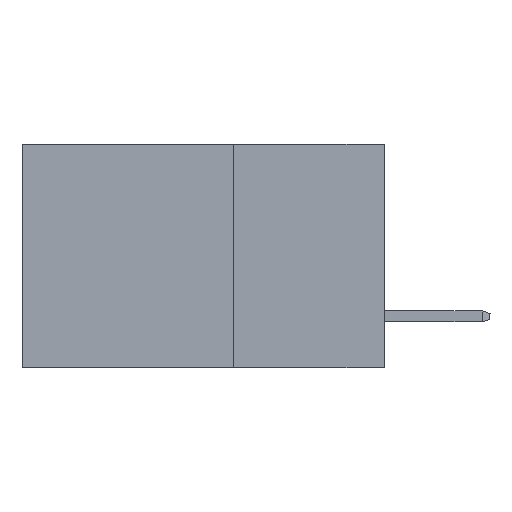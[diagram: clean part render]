
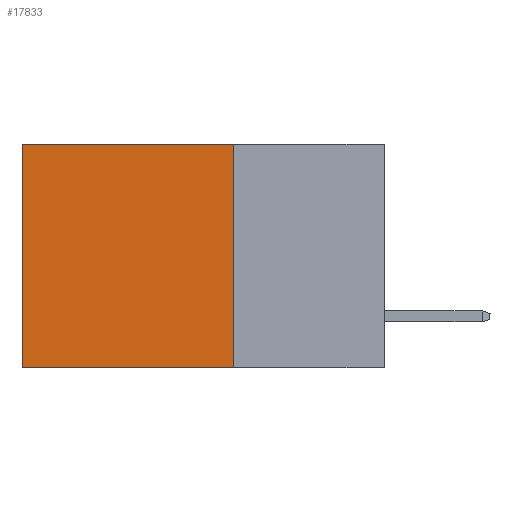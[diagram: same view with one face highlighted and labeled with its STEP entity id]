
A CAD part, left-side view. The second image highlights one B-rep face of the part: STEP entity #17833.
In plain terms, the highlighted planar face has unit normal (-1, 0, 0).
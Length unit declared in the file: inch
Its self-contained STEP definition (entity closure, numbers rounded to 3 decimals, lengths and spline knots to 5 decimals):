
#296 = DIRECTION ( 'NONE',  ( 0., 1., 0. ) ) ;
#643 = LINE ( 'NONE', #16362, #6996 ) ;
#756 = EDGE_CURVE ( 'NONE', #7188, #18939, #19447, .T. ) ;
#1616 = EDGE_LOOP ( 'NONE', ( #19284, #16431, #19518, #5918 ) ) ;
#2110 = VECTOR ( 'NONE', #296, 39.37008 ) ;
#2477 = EDGE_CURVE ( 'NONE', #15027, #7188, #20271, .T. ) ;
#3031 = DIRECTION ( 'NONE',  ( 1., 0., 0. ) ) ;
#3772 = LINE ( 'NONE', #13108, #18214 ) ;
#4811 = DIRECTION ( 'NONE',  ( 0., 0., -1. ) ) ;
#5918 = ORIENTED_EDGE ( 'NONE', *, *, #14782, .T. ) ;
#6092 = CARTESIAN_POINT ( 'NONE',  ( 0.2615, 0.25, -0.37 ) ) ;
#6996 = VECTOR ( 'NONE', #8333, 39.37008 ) ;
#7080 = VECTOR ( 'NONE', #15521, 39.37008 ) ;
#7188 = VERTEX_POINT ( 'NONE', #10137 ) ;
#8333 = DIRECTION ( 'NONE',  ( 0., 0., -1. ) ) ;
#10111 = DIRECTION ( 'NONE',  ( 0., 1., 0. ) ) ;
#10137 = CARTESIAN_POINT ( 'NONE',  ( 0.2615, 0.25, -0.37 ) ) ;
#11807 = CARTESIAN_POINT ( 'NONE',  ( 0.2615, 0.6, -0.37 ) ) ;
#12476 = CARTESIAN_POINT ( 'NONE',  ( 0.2615, 0.25, -0.37 ) ) ;
#12574 = PLANE ( 'NONE',  #13720 ) ;
#12859 = CARTESIAN_POINT ( 'NONE',  ( 0.2615, 0.6, 0. ) ) ;
#13108 = CARTESIAN_POINT ( 'NONE',  ( 0.2615, 0.25, 0. ) ) ;
#13620 = CARTESIAN_POINT ( 'NONE',  ( 0.2615, 0.25, 0. ) ) ;
#13720 = AXIS2_PLACEMENT_3D ( 'NONE', #12476, #3031, #4811 ) ;
#14025 = VERTEX_POINT ( 'NONE', #12859 ) ;
#14137 = FACE_OUTER_BOUND ( 'NONE', #1616, .T. ) ;
#14628 = EDGE_CURVE ( 'NONE', #14025, #18939, #643, .T. ) ;
#14782 = EDGE_CURVE ( 'NONE', #15027, #14025, #3772, .T. ) ;
#15027 = VERTEX_POINT ( 'NONE', #13620 ) ;
#15521 = DIRECTION ( 'NONE',  ( 0., 0., -1. ) ) ;
#16362 = CARTESIAN_POINT ( 'NONE',  ( 0.2615, 0.6, -0.37 ) ) ;
#16431 = ORIENTED_EDGE ( 'NONE', *, *, #756, .F. ) ;
#17677 = CARTESIAN_POINT ( 'NONE',  ( 0.2615, 0.25, -0.37 ) ) ;
#17833 = ADVANCED_FACE ( 'NONE', ( #14137 ), #12574, .F. ) ;
#18214 = VECTOR ( 'NONE', #10111, 39.37008 ) ;
#18939 = VERTEX_POINT ( 'NONE', #11807 ) ;
#19284 = ORIENTED_EDGE ( 'NONE', *, *, #14628, .T. ) ;
#19447 = LINE ( 'NONE', #17677, #2110 ) ;
#19518 = ORIENTED_EDGE ( 'NONE', *, *, #2477, .F. ) ;
#20271 = LINE ( 'NONE', #6092, #7080 ) ;
